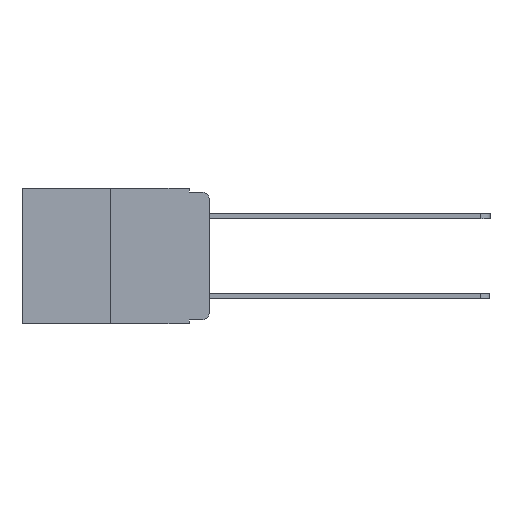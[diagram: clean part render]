
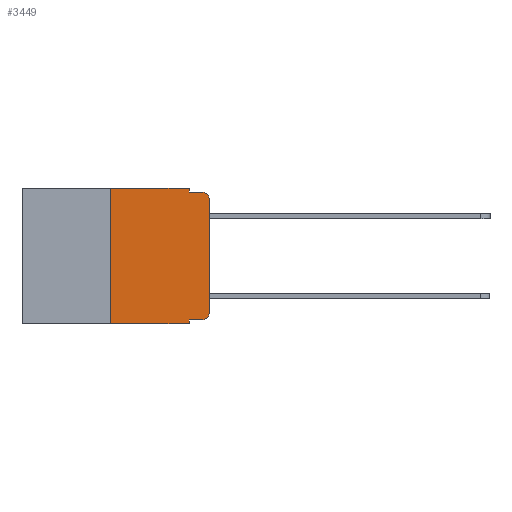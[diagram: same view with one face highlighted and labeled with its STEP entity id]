
A CAD part, left-side view. The second image highlights one B-rep face of the part: STEP entity #3449.
In plain terms, the highlighted planar face has unit normal (-1, 0, 0).
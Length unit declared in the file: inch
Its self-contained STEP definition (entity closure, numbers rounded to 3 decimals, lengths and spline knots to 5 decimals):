
#115 = CARTESIAN_POINT ( 'NONE',  ( 0., 0., 0. ) ) ;
#434 = EDGE_CURVE ( 'NONE', #6106, #5969, #12019, .T. ) ;
#475 = VERTEX_POINT ( 'NONE', #20093 ) ;
#608 = ORIENTED_EDGE ( 'NONE', *, *, #20027, .T. ) ;
#837 = CARTESIAN_POINT ( 'NONE',  ( 0., 0.473, -0.343 ) ) ;
#967 = EDGE_CURVE ( 'NONE', #5435, #475, #6262, .T. ) ;
#1327 = VERTEX_POINT ( 'NONE', #5548 ) ;
#1364 = DIRECTION ( 'NONE',  ( 0., 0., -1. ) ) ;
#1621 = CARTESIAN_POINT ( 'NONE',  ( 0., 0.473, 0. ) ) ;
#1718 = EDGE_CURVE ( 'NONE', #5435, #5969, #18580, .T. ) ;
#1925 = CARTESIAN_POINT ( 'NONE',  ( 0., 0.051, 0. ) ) ;
#1962 = VECTOR ( 'NONE', #15770, 39.37008 ) ;
#2498 = CIRCLE ( 'NONE', #7484, 0.02 ) ;
#2851 = EDGE_CURVE ( 'NONE', #6106, #1327, #14727, .T. ) ;
#3301 = DIRECTION ( 'NONE',  ( 0., 0., -1. ) ) ;
#3449 = ADVANCED_FACE ( 'NONE', ( #12311 ), #18556, .F. ) ;
#3610 = VECTOR ( 'NONE', #8046, 39.37008 ) ;
#4975 = EDGE_CURVE ( 'NONE', #17944, #18149, #6203, .T. ) ;
#5061 = ORIENTED_EDGE ( 'NONE', *, *, #4975, .F. ) ;
#5177 = AXIS2_PLACEMENT_3D ( 'NONE', #1621, #6434, #17079 ) ;
#5191 = CARTESIAN_POINT ( 'NONE',  ( 0., 0.051, -0.333 ) ) ;
#5316 = CIRCLE ( 'NONE', #20037, 0.02 ) ;
#5435 = VERTEX_POINT ( 'NONE', #16940 ) ;
#5548 = CARTESIAN_POINT ( 'NONE',  ( 0., 0.25, 0. ) ) ;
#5711 = ORIENTED_EDGE ( 'NONE', *, *, #7035, .F. ) ;
#5969 = VERTEX_POINT ( 'NONE', #12682 ) ;
#6106 = VERTEX_POINT ( 'NONE', #14473 ) ;
#6203 = LINE ( 'NONE', #1925, #1962 ) ;
#6262 = LINE ( 'NONE', #5191, #6730 ) ;
#6273 = CARTESIAN_POINT ( 'NONE',  ( 0., 0.051, 0. ) ) ;
#6434 = DIRECTION ( 'NONE',  ( 1., 0., 0. ) ) ;
#6730 = VECTOR ( 'NONE', #14324, 39.37008 ) ;
#6846 = CARTESIAN_POINT ( 'NONE',  ( 0., 0.02, -0.313 ) ) ;
#6916 = VECTOR ( 'NONE', #3301, 39.37008 ) ;
#7035 = EDGE_CURVE ( 'NONE', #18149, #7443, #13750, .T. ) ;
#7091 = VECTOR ( 'NONE', #8087, 39.37008 ) ;
#7443 = VERTEX_POINT ( 'NONE', #19817 ) ;
#7484 = AXIS2_PLACEMENT_3D ( 'NONE', #6846, #17489, #8386 ) ;
#7969 = VECTOR ( 'NONE', #18031, 39.37008 ) ;
#7971 = ORIENTED_EDGE ( 'NONE', *, *, #1718, .F. ) ;
#8046 = DIRECTION ( 'NONE',  ( 0., -1., 0. ) ) ;
#8087 = DIRECTION ( 'NONE',  ( 0., 0., 1. ) ) ;
#8325 = ORIENTED_EDGE ( 'NONE', *, *, #16628, .F. ) ;
#8386 = DIRECTION ( 'NONE',  ( 0., 0., -1. ) ) ;
#8456 = ORIENTED_EDGE ( 'NONE', *, *, #967, .T. ) ;
#9131 = ORIENTED_EDGE ( 'NONE', *, *, #13161, .T. ) ;
#9425 = ORIENTED_EDGE ( 'NONE', *, *, #434, .T. ) ;
#9684 = VECTOR ( 'NONE', #17622, 39.37008 ) ;
#9704 = DIRECTION ( 'NONE',  ( 0., 0., 1. ) ) ;
#10559 = CARTESIAN_POINT ( 'NONE',  ( 0., 0., -0.313 ) ) ;
#10562 = VERTEX_POINT ( 'NONE', #17424 ) ;
#10707 = ORIENTED_EDGE ( 'NONE', *, *, #12143, .T. ) ;
#10756 = DIRECTION ( 'NONE',  ( -1., 0., 0. ) ) ;
#10769 = VECTOR ( 'NONE', #9704, 39.37008 ) ;
#11815 = LINE ( 'NONE', #17158, #3610 ) ;
#12019 = LINE ( 'NONE', #837, #7969 ) ;
#12024 = VERTEX_POINT ( 'NONE', #10559 ) ;
#12143 = EDGE_CURVE ( 'NONE', #10562, #7443, #5316, .T. ) ;
#12311 = FACE_OUTER_BOUND ( 'NONE', #19082, .T. ) ;
#12524 = CARTESIAN_POINT ( 'NONE',  ( 0., 0.051, 0. ) ) ;
#12682 = CARTESIAN_POINT ( 'NONE',  ( 0., 0.051, -0.343 ) ) ;
#13161 = EDGE_CURVE ( 'NONE', #12024, #10562, #14830, .T. ) ;
#13750 = LINE ( 'NONE', #16094, #9684 ) ;
#14261 = CARTESIAN_POINT ( 'NONE',  ( 0., 0.051, -0.01 ) ) ;
#14324 = DIRECTION ( 'NONE',  ( 0., -1., 0. ) ) ;
#14473 = CARTESIAN_POINT ( 'NONE',  ( 0., 0.25, -0.343 ) ) ;
#14727 = LINE ( 'NONE', #17190, #7091 ) ;
#14830 = LINE ( 'NONE', #115, #10769 ) ;
#15770 = DIRECTION ( 'NONE',  ( 0., 0., -1. ) ) ;
#16094 = CARTESIAN_POINT ( 'NONE',  ( 0., 0.051, -0.01 ) ) ;
#16628 = EDGE_CURVE ( 'NONE', #1327, #17944, #11815, .T. ) ;
#16940 = CARTESIAN_POINT ( 'NONE',  ( 0., 0.051, -0.333 ) ) ;
#17079 = DIRECTION ( 'NONE',  ( 0., 0., -1. ) ) ;
#17158 = CARTESIAN_POINT ( 'NONE',  ( 0., 0.473, 0. ) ) ;
#17190 = CARTESIAN_POINT ( 'NONE',  ( 0., 0.25, 0. ) ) ;
#17424 = CARTESIAN_POINT ( 'NONE',  ( 0., 0., -0.03 ) ) ;
#17489 = DIRECTION ( 'NONE',  ( -1., 0., 0. ) ) ;
#17622 = DIRECTION ( 'NONE',  ( 0., -1., 0. ) ) ;
#17820 = ORIENTED_EDGE ( 'NONE', *, *, #2851, .F. ) ;
#17944 = VERTEX_POINT ( 'NONE', #6273 ) ;
#18031 = DIRECTION ( 'NONE',  ( 0., -1., 0. ) ) ;
#18149 = VERTEX_POINT ( 'NONE', #14261 ) ;
#18556 = PLANE ( 'NONE',  #5177 ) ;
#18580 = LINE ( 'NONE', #12524, #6916 ) ;
#19082 = EDGE_LOOP ( 'NONE', ( #9131, #10707, #5711, #5061, #8325, #17820, #9425, #7971, #8456, #608 ) ) ;
#19817 = CARTESIAN_POINT ( 'NONE',  ( 0., 0.02, -0.01 ) ) ;
#19862 = CARTESIAN_POINT ( 'NONE',  ( 0., 0.02, -0.03 ) ) ;
#20027 = EDGE_CURVE ( 'NONE', #475, #12024, #2498, .T. ) ;
#20037 = AXIS2_PLACEMENT_3D ( 'NONE', #19862, #10756, #1364 ) ;
#20093 = CARTESIAN_POINT ( 'NONE',  ( 0., 0.02, -0.333 ) ) ;
